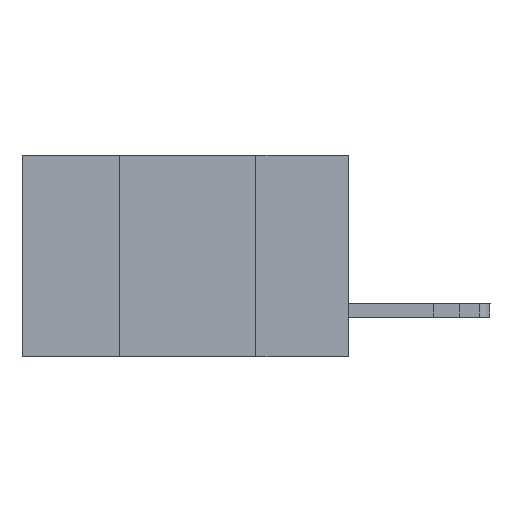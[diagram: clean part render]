
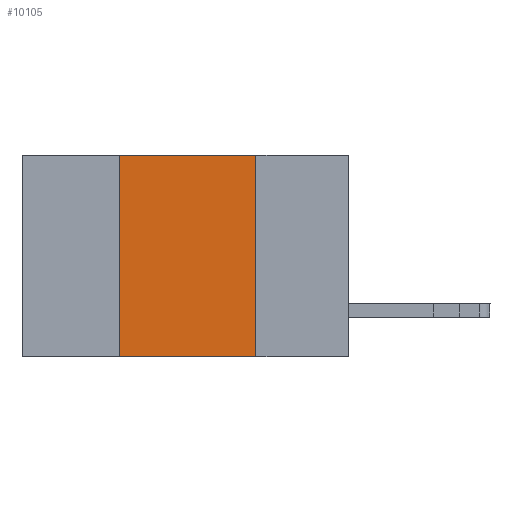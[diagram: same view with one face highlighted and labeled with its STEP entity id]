
A CAD part, left-side view. The second image highlights one B-rep face of the part: STEP entity #10105.
In plain terms, the highlighted planar face has unit normal (-1, 0, 0).
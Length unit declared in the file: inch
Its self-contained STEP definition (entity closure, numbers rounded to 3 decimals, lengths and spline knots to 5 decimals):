
#345 = CARTESIAN_POINT ( 'NONE',  ( 0., 0.17, 0. ) ) ;
#658 = VECTOR ( 'NONE', #12365, 39.37008 ) ;
#662 = LINE ( 'NONE', #8838, #658 ) ;
#1127 = VERTEX_POINT ( 'NONE', #2560 ) ;
#2293 = DIRECTION ( 'NONE',  ( 0., -1., 0. ) ) ;
#2489 = EDGE_CURVE ( 'NONE', #13766, #1127, #662, .T. ) ;
#2560 = CARTESIAN_POINT ( 'NONE',  ( 0., 0.42, 0. ) ) ;
#4024 = VERTEX_POINT ( 'NONE', #9208 ) ;
#4223 = LINE ( 'NONE', #4296, #14413 ) ;
#4296 = CARTESIAN_POINT ( 'NONE',  ( 0., 0.6, -0.37 ) ) ;
#5207 = FACE_OUTER_BOUND ( 'NONE', #8501, .T. ) ;
#5716 = CARTESIAN_POINT ( 'NONE',  ( 0., 0.6, 0. ) ) ;
#6537 = AXIS2_PLACEMENT_3D ( 'NONE', #7522, #7689, #10146 ) ;
#6594 = DIRECTION ( 'NONE',  ( 0., 0., -1. ) ) ;
#6874 = LINE ( 'NONE', #5716, #9506 ) ;
#7286 = VECTOR ( 'NONE', #6594, 39.37008 ) ;
#7522 = CARTESIAN_POINT ( 'NONE',  ( 0., 0.6, 0. ) ) ;
#7689 = DIRECTION ( 'NONE',  ( 1., 0., 0. ) ) ;
#8144 = ORIENTED_EDGE ( 'NONE', *, *, #2489, .F. ) ;
#8323 = ORIENTED_EDGE ( 'NONE', *, *, #11345, .F. ) ;
#8501 = EDGE_LOOP ( 'NONE', ( #8323, #9632, #8144, #14602 ) ) ;
#8838 = CARTESIAN_POINT ( 'NONE',  ( 0., 0.42, -0.37 ) ) ;
#8896 = DIRECTION ( 'NONE',  ( 0., -1., 0. ) ) ;
#8988 = CARTESIAN_POINT ( 'NONE',  ( 0., 0.17, -0.37 ) ) ;
#9149 = EDGE_CURVE ( 'NONE', #1127, #13291, #6874, .T. ) ;
#9208 = CARTESIAN_POINT ( 'NONE',  ( 0., 0.17, -0.37 ) ) ;
#9506 = VECTOR ( 'NONE', #2293, 39.37008 ) ;
#9632 = ORIENTED_EDGE ( 'NONE', *, *, #9149, .F. ) ;
#10105 = ADVANCED_FACE ( 'NONE', ( #5207 ), #13528, .F. ) ;
#10146 = DIRECTION ( 'NONE',  ( 0., 0., -1. ) ) ;
#11345 = EDGE_CURVE ( 'NONE', #13291, #4024, #14577, .T. ) ;
#11547 = CARTESIAN_POINT ( 'NONE',  ( 0., 0.42, -0.37 ) ) ;
#11812 = EDGE_CURVE ( 'NONE', #13766, #4024, #4223, .T. ) ;
#12365 = DIRECTION ( 'NONE',  ( 0., 0., 1. ) ) ;
#13291 = VERTEX_POINT ( 'NONE', #345 ) ;
#13528 = PLANE ( 'NONE',  #6537 ) ;
#13766 = VERTEX_POINT ( 'NONE', #11547 ) ;
#14413 = VECTOR ( 'NONE', #8896, 39.37008 ) ;
#14577 = LINE ( 'NONE', #8988, #7286 ) ;
#14602 = ORIENTED_EDGE ( 'NONE', *, *, #11812, .T. ) ;
